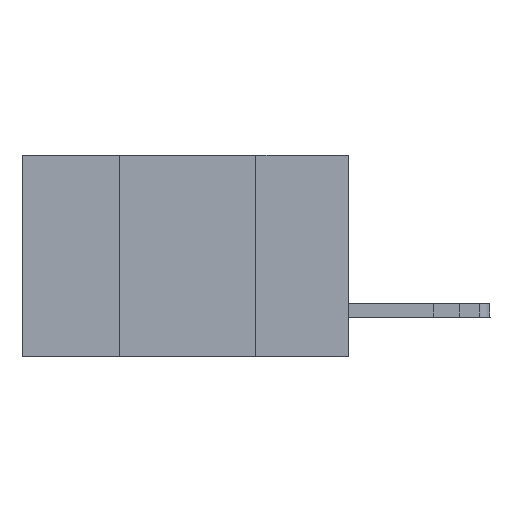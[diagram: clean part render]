
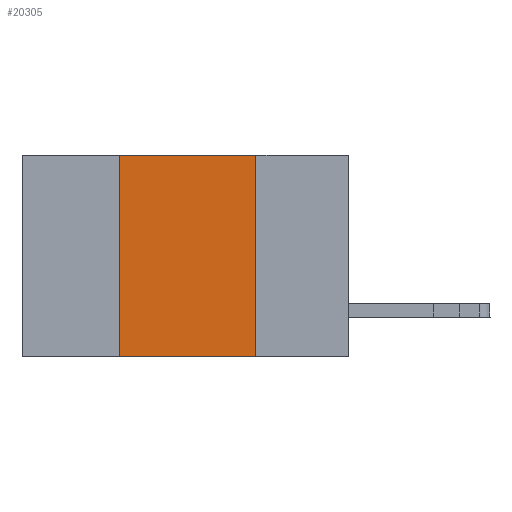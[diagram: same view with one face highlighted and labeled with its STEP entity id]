
A CAD part, left-side view. The second image highlights one B-rep face of the part: STEP entity #20305.
In plain terms, the highlighted planar face has unit normal (-1, 0, 0).
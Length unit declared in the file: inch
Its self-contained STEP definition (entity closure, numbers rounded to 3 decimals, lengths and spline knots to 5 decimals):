
#518 = DIRECTION ( 'NONE',  ( 0., -1., 0. ) ) ;
#1765 = CARTESIAN_POINT ( 'NONE',  ( 0., 0.42, 0. ) ) ;
#2913 = ORIENTED_EDGE ( 'NONE', *, *, #18316, .F. ) ;
#3254 = VECTOR ( 'NONE', #7381, 39.37008 ) ;
#3565 = DIRECTION ( 'NONE',  ( 0., -1., 0. ) ) ;
#3739 = ORIENTED_EDGE ( 'NONE', *, *, #8550, .T. ) ;
#4167 = LINE ( 'NONE', #9715, #22889 ) ;
#4825 = VECTOR ( 'NONE', #3565, 39.37008 ) ;
#5511 = DIRECTION ( 'NONE',  ( 1., 0., 0. ) ) ;
#5672 = CARTESIAN_POINT ( 'NONE',  ( 0., 0.42, 0. ) ) ;
#7043 = EDGE_CURVE ( 'NONE', #14411, #23008, #4167, .T. ) ;
#7381 = DIRECTION ( 'NONE',  ( 0., 0., 1. ) ) ;
#7607 = LINE ( 'NONE', #5672, #3254 ) ;
#7673 = DIRECTION ( 'NONE',  ( 0., 0., -1. ) ) ;
#8423 = LINE ( 'NONE', #11946, #9441 ) ;
#8550 = EDGE_CURVE ( 'NONE', #19004, #18665, #14575, .T. ) ;
#9441 = VECTOR ( 'NONE', #10105, 39.37008 ) ;
#9715 = CARTESIAN_POINT ( 'NONE',  ( 0., 0.6, 0. ) ) ;
#10105 = DIRECTION ( 'NONE',  ( 0., 0., -1. ) ) ;
#10504 = EDGE_CURVE ( 'NONE', #19004, #14411, #7607, .T. ) ;
#10864 = CARTESIAN_POINT ( 'NONE',  ( 0., 0.17, 0. ) ) ;
#11946 = CARTESIAN_POINT ( 'NONE',  ( 0., 0.17, 0. ) ) ;
#13832 = ORIENTED_EDGE ( 'NONE', *, *, #7043, .F. ) ;
#14063 = ORIENTED_EDGE ( 'NONE', *, *, #10504, .F. ) ;
#14411 = VERTEX_POINT ( 'NONE', #1765 ) ;
#14575 = LINE ( 'NONE', #20139, #4825 ) ;
#16389 = PLANE ( 'NONE',  #22249 ) ;
#17360 = CARTESIAN_POINT ( 'NONE',  ( 0., 0.17, -0.37 ) ) ;
#17832 = EDGE_LOOP ( 'NONE', ( #2913, #13832, #14063, #3739 ) ) ;
#18316 = EDGE_CURVE ( 'NONE', #23008, #18665, #8423, .T. ) ;
#18665 = VERTEX_POINT ( 'NONE', #17360 ) ;
#19004 = VERTEX_POINT ( 'NONE', #20482 ) ;
#20139 = CARTESIAN_POINT ( 'NONE',  ( 0., 0.6, -0.37 ) ) ;
#20143 = FACE_OUTER_BOUND ( 'NONE', #17832, .T. ) ;
#20305 = ADVANCED_FACE ( 'NONE', ( #20143 ), #16389, .F. ) ;
#20370 = CARTESIAN_POINT ( 'NONE',  ( 0., 0.6, 0. ) ) ;
#20482 = CARTESIAN_POINT ( 'NONE',  ( 0., 0.42, -0.37 ) ) ;
#22249 = AXIS2_PLACEMENT_3D ( 'NONE', #20370, #5511, #7673 ) ;
#22889 = VECTOR ( 'NONE', #518, 39.37008 ) ;
#23008 = VERTEX_POINT ( 'NONE', #10864 ) ;
